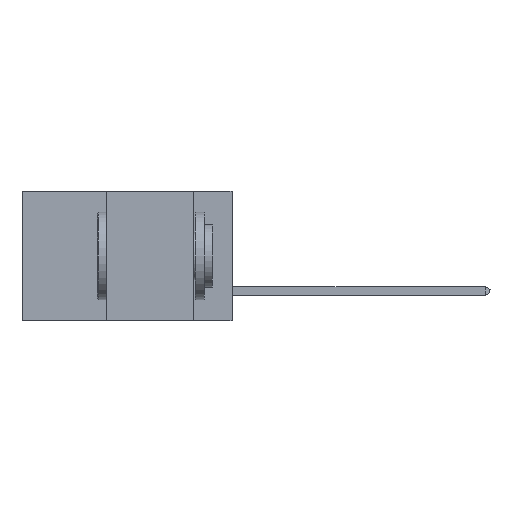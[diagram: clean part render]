
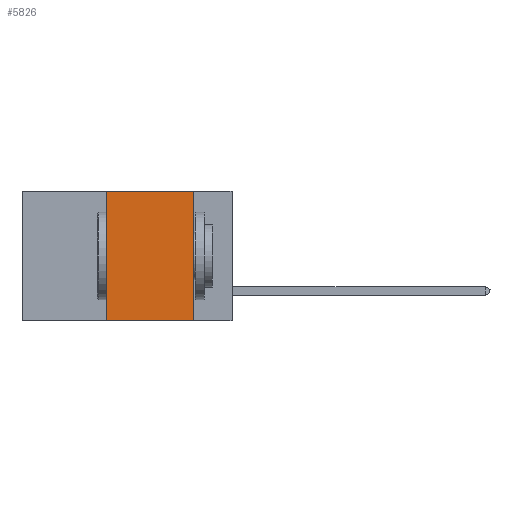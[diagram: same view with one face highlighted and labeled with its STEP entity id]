
A CAD part, left-side view. The second image highlights one B-rep face of the part: STEP entity #5826.
In plain terms, the highlighted planar face has unit normal (-1, 0, 0).
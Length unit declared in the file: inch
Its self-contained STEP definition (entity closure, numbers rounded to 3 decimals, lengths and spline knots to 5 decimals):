
#243 = DIRECTION ( 'NONE',  ( 0., -1., 0. ) ) ;
#739 = VECTOR ( 'NONE', #3823, 39.37008 ) ;
#1041 = CARTESIAN_POINT ( 'NONE',  ( 0., 0.36, 0. ) ) ;
#1748 = DIRECTION ( 'NONE',  ( 0., 0., -1. ) ) ;
#2300 = CARTESIAN_POINT ( 'NONE',  ( 0., 0.36, 0. ) ) ;
#2744 = PLANE ( 'NONE',  #7551 ) ;
#3138 = ORIENTED_EDGE ( 'NONE', *, *, #12431, .T. ) ;
#3237 = CARTESIAN_POINT ( 'NONE',  ( 0., 0.6, 0. ) ) ;
#3796 = EDGE_CURVE ( 'NONE', #10364, #12379, #7872, .T. ) ;
#3823 = DIRECTION ( 'NONE',  ( 0., -1., 0. ) ) ;
#3907 = LINE ( 'NONE', #3237, #4401 ) ;
#4267 = EDGE_LOOP ( 'NONE', ( #8662, #7887, #8037, #3138 ) ) ;
#4401 = VECTOR ( 'NONE', #243, 39.37008 ) ;
#5047 = VECTOR ( 'NONE', #8050, 39.37008 ) ;
#5802 = LINE ( 'NONE', #2300, #8634 ) ;
#5826 = ADVANCED_FACE ( 'NONE', ( #8418 ), #2744, .F. ) ;
#6812 = CARTESIAN_POINT ( 'NONE',  ( 0., 0.6, 0. ) ) ;
#7535 = CARTESIAN_POINT ( 'NONE',  ( 0., 0.11, 0. ) ) ;
#7551 = AXIS2_PLACEMENT_3D ( 'NONE', #6812, #7831, #1748 ) ;
#7831 = DIRECTION ( 'NONE',  ( 1., 0., 0. ) ) ;
#7872 = LINE ( 'NONE', #8092, #5047 ) ;
#7887 = ORIENTED_EDGE ( 'NONE', *, *, #12133, .F. ) ;
#8037 = ORIENTED_EDGE ( 'NONE', *, *, #9810, .F. ) ;
#8050 = DIRECTION ( 'NONE',  ( 0., 0., -1. ) ) ;
#8092 = CARTESIAN_POINT ( 'NONE',  ( 0., 0.11, 0. ) ) ;
#8418 = FACE_OUTER_BOUND ( 'NONE', #4267, .T. ) ;
#8634 = VECTOR ( 'NONE', #10349, 39.37008 ) ;
#8662 = ORIENTED_EDGE ( 'NONE', *, *, #3796, .F. ) ;
#9360 = VERTEX_POINT ( 'NONE', #12929 ) ;
#9810 = EDGE_CURVE ( 'NONE', #9360, #10170, #5802, .T. ) ;
#10170 = VERTEX_POINT ( 'NONE', #1041 ) ;
#10349 = DIRECTION ( 'NONE',  ( 0., 0., 1. ) ) ;
#10364 = VERTEX_POINT ( 'NONE', #7535 ) ;
#11938 = LINE ( 'NONE', #12905, #739 ) ;
#12133 = EDGE_CURVE ( 'NONE', #10170, #10364, #3907, .T. ) ;
#12379 = VERTEX_POINT ( 'NONE', #12696 ) ;
#12431 = EDGE_CURVE ( 'NONE', #9360, #12379, #11938, .T. ) ;
#12696 = CARTESIAN_POINT ( 'NONE',  ( 0., 0.11, -0.37 ) ) ;
#12905 = CARTESIAN_POINT ( 'NONE',  ( 0., 0.6, -0.37 ) ) ;
#12929 = CARTESIAN_POINT ( 'NONE',  ( 0., 0.36, -0.37 ) ) ;
